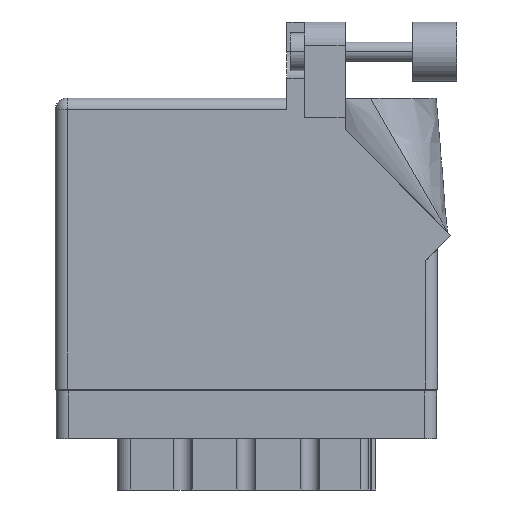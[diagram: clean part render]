
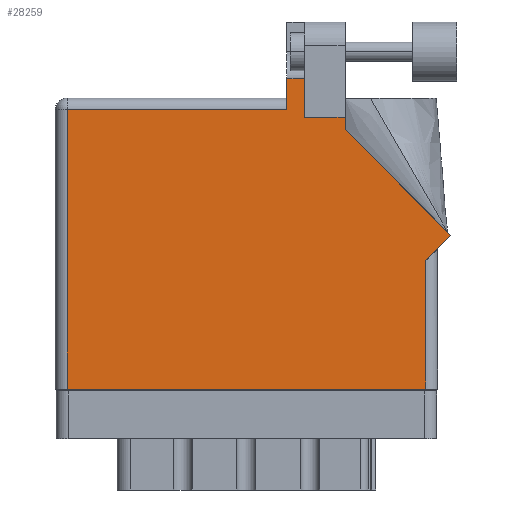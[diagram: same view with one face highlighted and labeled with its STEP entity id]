
A CAD part, front view. The second image highlights one B-rep face of the part: STEP entity #28259.
In plain terms, the highlighted face is planar.
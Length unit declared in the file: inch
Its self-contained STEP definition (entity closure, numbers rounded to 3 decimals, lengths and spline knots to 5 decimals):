
#727 = DIRECTION ( 'NONE',  ( 0., 1., 0. ) ) ;
#1155 = CARTESIAN_POINT ( 'NONE',  ( 2.08071, 0.80771, 0. ) ) ;
#1279 = DIRECTION ( 'NONE',  ( 0., 0., -1. ) ) ;
#1463 = EDGE_CURVE ( 'NONE', #4607, #8084, #30784, .T. ) ;
#1860 = ORIENTED_EDGE ( 'NONE', *, *, #15214, .T. ) ;
#3177 = VECTOR ( 'NONE', #20429, 39.37008 ) ;
#3443 = VECTOR ( 'NONE', #31470, 39.37008 ) ;
#3950 = PLANE ( 'NONE',  #9234 ) ;
#4208 = CARTESIAN_POINT ( 'NONE',  ( 1.64177, 1.6315, 0. ) ) ;
#4228 = VECTOR ( 'NONE', #28377, 39.37008 ) ;
#4607 = VERTEX_POINT ( 'NONE', #11999 ) ;
#4887 = CARTESIAN_POINT ( 'NONE',  ( 0.062, 0., 0. ) ) ;
#4936 = LINE ( 'NONE', #15159, #3443 ) ;
#5259 = ORIENTED_EDGE ( 'NONE', *, *, #19849, .T. ) ;
#5320 = ORIENTED_EDGE ( 'NONE', *, *, #31717, .T. ) ;
#5432 = LINE ( 'NONE', #7954, #20438 ) ;
#5730 = CARTESIAN_POINT ( 'NONE',  ( 1.948, 0., 0. ) ) ;
#6097 = ORIENTED_EDGE ( 'NONE', *, *, #1463, .T. ) ;
#6798 = EDGE_CURVE ( 'NONE', #40297, #4607, #25319, .T. ) ;
#7176 = VERTEX_POINT ( 'NONE', #5730 ) ;
#7743 = VECTOR ( 'NONE', #21176, 39.37008 ) ;
#7806 = DIRECTION ( 'NONE',  ( -1., 0., 0. ) ) ;
#7894 = CARTESIAN_POINT ( 'NONE',  ( 1.217, 1.53, 0. ) ) ;
#7923 = CARTESIAN_POINT ( 'NONE',  ( 1.948, 0.675, 0. ) ) ;
#7954 = CARTESIAN_POINT ( 'NONE',  ( 1.524, 1.43, 0. ) ) ;
#8084 = VERTEX_POINT ( 'NONE', #24919 ) ;
#8086 = ORIENTED_EDGE ( 'NONE', *, *, #6798, .T. ) ;
#8284 = CARTESIAN_POINT ( 'NONE',  ( 2.08071, 0.80771, 0. ) ) ;
#8784 = ORIENTED_EDGE ( 'NONE', *, *, #32215, .T. ) ;
#9175 = LINE ( 'NONE', #4208, #3177 ) ;
#9234 = AXIS2_PLACEMENT_3D ( 'NONE', #20449, #1279, #23938 ) ;
#9909 = VERTEX_POINT ( 'NONE', #11589 ) ;
#11444 = EDGE_LOOP ( 'NONE', ( #1860, #26212, #8086, #6097, #5259, #11565, #13587, #5320, #8784, #36876, #31087 ) ) ;
#11565 = ORIENTED_EDGE ( 'NONE', *, *, #16202, .T. ) ;
#11589 = CARTESIAN_POINT ( 'NONE',  ( 1.524, 1.36442, 0. ) ) ;
#11943 = VERTEX_POINT ( 'NONE', #35773 ) ;
#11999 = CARTESIAN_POINT ( 'NONE',  ( 1.217, 1.468, 0. ) ) ;
#12200 = VECTOR ( 'NONE', #39899, 39.37008 ) ;
#12312 = CARTESIAN_POINT ( 'NONE',  ( 1.311, 1.6315, 0. ) ) ;
#13587 = ORIENTED_EDGE ( 'NONE', *, *, #20454, .T. ) ;
#13793 = CARTESIAN_POINT ( 'NONE',  ( 1.311, 1.43, 0. ) ) ;
#14000 = VERTEX_POINT ( 'NONE', #13793 ) ;
#15159 = CARTESIAN_POINT ( 'NONE',  ( 0., 0., 0. ) ) ;
#15214 = EDGE_CURVE ( 'NONE', #14000, #18777, #17037, .T. ) ;
#16202 = EDGE_CURVE ( 'NONE', #22914, #7176, #4936, .T. ) ;
#16867 = VERTEX_POINT ( 'NONE', #8284 ) ;
#17037 = LINE ( 'NONE', #22973, #27084 ) ;
#17996 = CARTESIAN_POINT ( 'NONE',  ( 1.524, 1.36442, 0. ) ) ;
#18144 = VECTOR ( 'NONE', #23252, 39.37008 ) ;
#18392 = CARTESIAN_POINT ( 'NONE',  ( 2.01, 0.737, 0. ) ) ;
#18711 = DIRECTION ( 'NONE',  ( -1., 0., 0. ) ) ;
#18716 = VECTOR ( 'NONE', #18711, 39.37008 ) ;
#18769 = VECTOR ( 'NONE', #40443, 39.37008 ) ;
#18777 = VERTEX_POINT ( 'NONE', #12312 ) ;
#19352 = EDGE_CURVE ( 'NONE', #9909, #11943, #36310, .T. ) ;
#19849 = EDGE_CURVE ( 'NONE', #8084, #22914, #20725, .T. ) ;
#20429 = DIRECTION ( 'NONE',  ( -1., 0., 0. ) ) ;
#20438 = VECTOR ( 'NONE', #7806, 39.37008 ) ;
#20449 = CARTESIAN_POINT ( 'NONE',  ( 0., 1.53, 0. ) ) ;
#20454 = EDGE_CURVE ( 'NONE', #7176, #22181, #21173, .T. ) ;
#20725 = LINE ( 'NONE', #4887, #12200 ) ;
#20878 = CARTESIAN_POINT ( 'NONE',  ( 0.062, 0., 0. ) ) ;
#21173 = LINE ( 'NONE', #33361, #18144 ) ;
#21176 = DIRECTION ( 'NONE',  ( 0., -1., 0. ) ) ;
#22181 = VERTEX_POINT ( 'NONE', #7923 ) ;
#22914 = VERTEX_POINT ( 'NONE', #20878 ) ;
#22973 = CARTESIAN_POINT ( 'NONE',  ( 1.311, 1.43, 0. ) ) ;
#23252 = DIRECTION ( 'NONE',  ( 0., 1., 0. ) ) ;
#23938 = DIRECTION ( 'NONE',  ( -1., 0., 0. ) ) ;
#24919 = CARTESIAN_POINT ( 'NONE',  ( 0.062, 1.468, 0. ) ) ;
#25319 = LINE ( 'NONE', #7894, #7743 ) ;
#25920 = EDGE_CURVE ( 'NONE', #18777, #40297, #9175, .T. ) ;
#26212 = ORIENTED_EDGE ( 'NONE', *, *, #25920, .T. ) ;
#27084 = VECTOR ( 'NONE', #727, 39.37008 ) ;
#27389 = FACE_OUTER_BOUND ( 'NONE', #11444, .T. ) ;
#28259 = ADVANCED_FACE ( 'NONE', ( #27389 ), #3950, .F. ) ;
#28377 = DIRECTION ( 'NONE',  ( 0.707, 0.707, 0. ) ) ;
#28901 = EDGE_CURVE ( 'NONE', #11943, #14000, #5432, .T. ) ;
#29514 = CARTESIAN_POINT ( 'NONE',  ( 1.217, 1.6315, 0. ) ) ;
#30784 = LINE ( 'NONE', #35128, #18716 ) ;
#31087 = ORIENTED_EDGE ( 'NONE', *, *, #28901, .T. ) ;
#31470 = DIRECTION ( 'NONE',  ( 1., 0., 0. ) ) ;
#31717 = EDGE_CURVE ( 'NONE', #22181, #16867, #38782, .T. ) ;
#32215 = EDGE_CURVE ( 'NONE', #16867, #9909, #39313, .T. ) ;
#33286 = VECTOR ( 'NONE', #39527, 39.37008 ) ;
#33361 = CARTESIAN_POINT ( 'NONE',  ( 1.948, 0.737, 0. ) ) ;
#35128 = CARTESIAN_POINT ( 'NONE',  ( 0., 1.468, 0. ) ) ;
#35773 = CARTESIAN_POINT ( 'NONE',  ( 1.524, 1.43, 0. ) ) ;
#36310 = LINE ( 'NONE', #17996, #18769 ) ;
#36876 = ORIENTED_EDGE ( 'NONE', *, *, #19352, .T. ) ;
#38782 = LINE ( 'NONE', #18392, #4228 ) ;
#39313 = LINE ( 'NONE', #1155, #33286 ) ;
#39527 = DIRECTION ( 'NONE',  ( -0.707, 0.707, 0. ) ) ;
#39899 = DIRECTION ( 'NONE',  ( 0., -1., 0. ) ) ;
#40297 = VERTEX_POINT ( 'NONE', #29514 ) ;
#40443 = DIRECTION ( 'NONE',  ( 0., 1., 0. ) ) ;
